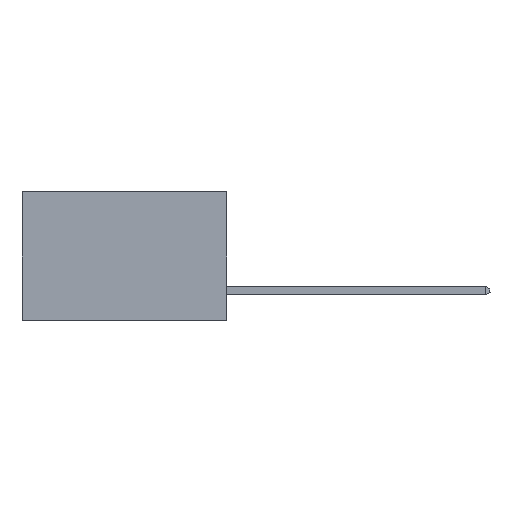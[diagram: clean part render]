
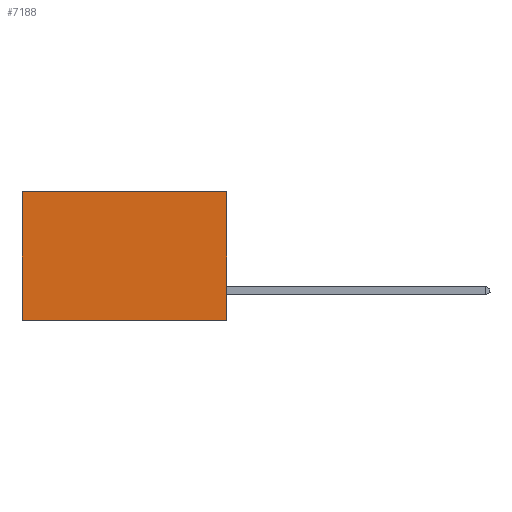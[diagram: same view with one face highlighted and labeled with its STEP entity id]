
A CAD part, left-side view. The second image highlights one B-rep face of the part: STEP entity #7188.
In plain terms, the highlighted planar face has unit normal (-1, 0, 0).
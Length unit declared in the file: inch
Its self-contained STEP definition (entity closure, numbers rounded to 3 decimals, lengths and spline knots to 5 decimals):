
#175 = EDGE_CURVE ( 'NONE', #9459, #3696, #14470, .T. ) ;
#217 = LINE ( 'NONE', #6939, #9532 ) ;
#237 = EDGE_CURVE ( 'NONE', #2983, #9459, #217, .T. ) ;
#745 = VECTOR ( 'NONE', #19960, 39.37008 ) ;
#799 = FACE_OUTER_BOUND ( 'NONE', #5063, .T. ) ;
#1288 = CARTESIAN_POINT ( 'NONE',  ( 0.277, 0., 0. ) ) ;
#1740 = ORIENTED_EDGE ( 'NONE', *, *, #19012, .T. ) ;
#2983 = VERTEX_POINT ( 'NONE', #1288 ) ;
#3392 = ORIENTED_EDGE ( 'NONE', *, *, #175, .F. ) ;
#3696 = VERTEX_POINT ( 'NONE', #20220 ) ;
#4054 = EDGE_CURVE ( 'NONE', #16407, #3696, #11799, .T. ) ;
#5063 = EDGE_LOOP ( 'NONE', ( #10862, #3392, #11400, #1740 ) ) ;
#6061 = DIRECTION ( 'NONE',  ( 0., 0., -1. ) ) ;
#6109 = DIRECTION ( 'NONE',  ( 1., 0., 0. ) ) ;
#6141 = PLANE ( 'NONE',  #8707 ) ;
#6293 = CARTESIAN_POINT ( 'NONE',  ( 0.277, 0., -0.37 ) ) ;
#6723 = DIRECTION ( 'NONE',  ( 0., 0., -1. ) ) ;
#6939 = CARTESIAN_POINT ( 'NONE',  ( 0.277, 0., -0.37 ) ) ;
#6985 = CARTESIAN_POINT ( 'NONE',  ( 0.277, 0.59, -0.37 ) ) ;
#7188 = ADVANCED_FACE ( 'NONE', ( #799 ), #6141, .F. ) ;
#8707 = AXIS2_PLACEMENT_3D ( 'NONE', #6293, #6109, #6061 ) ;
#9306 = DIRECTION ( 'NONE',  ( 0., 0., -1. ) ) ;
#9459 = VERTEX_POINT ( 'NONE', #17203 ) ;
#9532 = VECTOR ( 'NONE', #9306, 39.37008 ) ;
#10021 = LINE ( 'NONE', #11767, #745 ) ;
#10862 = ORIENTED_EDGE ( 'NONE', *, *, #4054, .T. ) ;
#11279 = VECTOR ( 'NONE', #6723, 39.37008 ) ;
#11400 = ORIENTED_EDGE ( 'NONE', *, *, #237, .F. ) ;
#11767 = CARTESIAN_POINT ( 'NONE',  ( 0.277, 0., 0. ) ) ;
#11799 = LINE ( 'NONE', #6985, #11279 ) ;
#14470 = LINE ( 'NONE', #17845, #14986 ) ;
#14986 = VECTOR ( 'NONE', #18038, 39.37008 ) ;
#16407 = VERTEX_POINT ( 'NONE', #19010 ) ;
#17203 = CARTESIAN_POINT ( 'NONE',  ( 0.277, 0., -0.37 ) ) ;
#17845 = CARTESIAN_POINT ( 'NONE',  ( 0.277, 0., -0.37 ) ) ;
#18038 = DIRECTION ( 'NONE',  ( 0., 1., 0. ) ) ;
#19010 = CARTESIAN_POINT ( 'NONE',  ( 0.277, 0.59, 0. ) ) ;
#19012 = EDGE_CURVE ( 'NONE', #2983, #16407, #10021, .T. ) ;
#19960 = DIRECTION ( 'NONE',  ( 0., 1., 0. ) ) ;
#20220 = CARTESIAN_POINT ( 'NONE',  ( 0.277, 0.59, -0.37 ) ) ;
